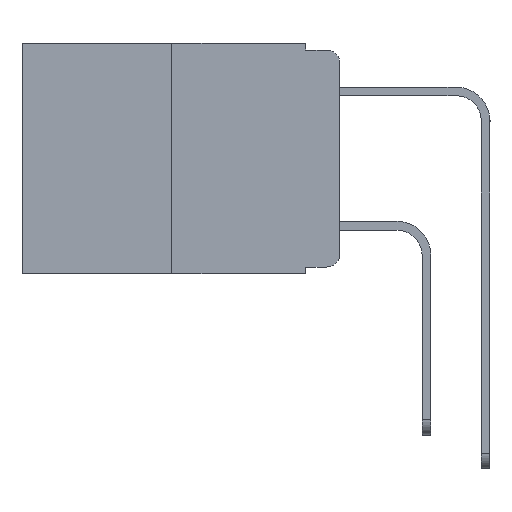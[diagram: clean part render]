
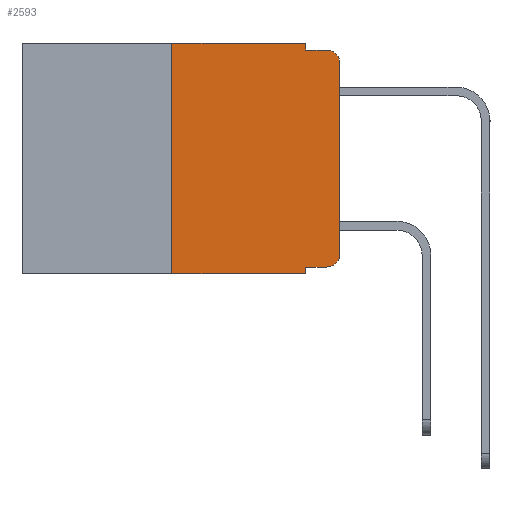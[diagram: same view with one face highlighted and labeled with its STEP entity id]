
A CAD part, left-side view. The second image highlights one B-rep face of the part: STEP entity #2593.
In plain terms, the highlighted planar face has unit normal (-1, 0, 0).
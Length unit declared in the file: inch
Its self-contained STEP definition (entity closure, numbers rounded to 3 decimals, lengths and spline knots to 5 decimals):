
#472 = CARTESIAN_POINT ( 'NONE',  ( 0., 0.051, 0. ) ) ;
#910 = EDGE_CURVE ( 'NONE', #5153, #4591, #5345, .T. ) ;
#1069 = VERTEX_POINT ( 'NONE', #21853 ) ;
#1688 = LINE ( 'NONE', #14134, #5685 ) ;
#1871 = CARTESIAN_POINT ( 'NONE',  ( 0., 0.25, -0.343 ) ) ;
#2239 = CARTESIAN_POINT ( 'NONE',  ( 0., 0.02, -0.313 ) ) ;
#2593 = ADVANCED_FACE ( 'NONE', ( #4491 ), #8141, .F. ) ;
#2603 = CARTESIAN_POINT ( 'NONE',  ( 0., 0.02, -0.333 ) ) ;
#2644 = VECTOR ( 'NONE', #14278, 39.37008 ) ;
#2890 = DIRECTION ( 'NONE',  ( 0., 0., -1. ) ) ;
#3186 = DIRECTION ( 'NONE',  ( 1., 0., 0. ) ) ;
#3280 = CARTESIAN_POINT ( 'NONE',  ( 0., 0.473, 0. ) ) ;
#3556 = DIRECTION ( 'NONE',  ( 0., -1., 0. ) ) ;
#3563 = EDGE_CURVE ( 'NONE', #10278, #11799, #20901, .T. ) ;
#3988 = DIRECTION ( 'NONE',  ( 0., 0., -1. ) ) ;
#4409 = EDGE_CURVE ( 'NONE', #4591, #10471, #15972, .T. ) ;
#4491 = FACE_OUTER_BOUND ( 'NONE', #20699, .T. ) ;
#4536 = CARTESIAN_POINT ( 'NONE',  ( 0., 0.473, -0.343 ) ) ;
#4591 = VERTEX_POINT ( 'NONE', #21033 ) ;
#5025 = CARTESIAN_POINT ( 'NONE',  ( 0., 0.02, -0.03 ) ) ;
#5153 = VERTEX_POINT ( 'NONE', #12522 ) ;
#5345 = LINE ( 'NONE', #20466, #17863 ) ;
#5370 = CARTESIAN_POINT ( 'NONE',  ( 0., 0.051, -0.01 ) ) ;
#5516 = EDGE_CURVE ( 'NONE', #16894, #10471, #6558, .T. ) ;
#5617 = CARTESIAN_POINT ( 'NONE',  ( 0., 0., -0.313 ) ) ;
#5626 = DIRECTION ( 'NONE',  ( 0., 0., 1. ) ) ;
#5685 = VECTOR ( 'NONE', #5626, 39.37008 ) ;
#6232 = VECTOR ( 'NONE', #7541, 39.37008 ) ;
#6558 = CIRCLE ( 'NONE', #13727, 0.02 ) ;
#6663 = EDGE_CURVE ( 'NONE', #15615, #16894, #15861, .T. ) ;
#6730 = DIRECTION ( 'NONE',  ( 0., 0., -1. ) ) ;
#7088 = CIRCLE ( 'NONE', #12472, 0.02 ) ;
#7541 = DIRECTION ( 'NONE',  ( 0., 0., 1. ) ) ;
#8141 = PLANE ( 'NONE',  #17940 ) ;
#8208 = LINE ( 'NONE', #13750, #17285 ) ;
#9211 = VERTEX_POINT ( 'NONE', #2603 ) ;
#9661 = DIRECTION ( 'NONE',  ( 0., -1., 0. ) ) ;
#10278 = VERTEX_POINT ( 'NONE', #1871 ) ;
#10471 = VERTEX_POINT ( 'NONE', #15963 ) ;
#10676 = CARTESIAN_POINT ( 'NONE',  ( 0., 0.25, 0. ) ) ;
#11799 = VERTEX_POINT ( 'NONE', #21342 ) ;
#12472 = AXIS2_PLACEMENT_3D ( 'NONE', #2239, #14167, #3988 ) ;
#12522 = CARTESIAN_POINT ( 'NONE',  ( 0., 0.051, 0. ) ) ;
#12553 = ORIENTED_EDGE ( 'NONE', *, *, #4409, .F. ) ;
#12594 = CARTESIAN_POINT ( 'NONE',  ( 0., 0.473, 0. ) ) ;
#12875 = ORIENTED_EDGE ( 'NONE', *, *, #21837, .F. ) ;
#13337 = ORIENTED_EDGE ( 'NONE', *, *, #5516, .T. ) ;
#13469 = ORIENTED_EDGE ( 'NONE', *, *, #14835, .F. ) ;
#13706 = ORIENTED_EDGE ( 'NONE', *, *, #3563, .T. ) ;
#13727 = AXIS2_PLACEMENT_3D ( 'NONE', #5025, #16941, #6730 ) ;
#13750 = CARTESIAN_POINT ( 'NONE',  ( 0., 0.051, -0.333 ) ) ;
#13885 = DIRECTION ( 'NONE',  ( 0., -1., 0. ) ) ;
#14134 = CARTESIAN_POINT ( 'NONE',  ( 0., 0.25, 0. ) ) ;
#14155 = ORIENTED_EDGE ( 'NONE', *, *, #910, .F. ) ;
#14167 = DIRECTION ( 'NONE',  ( -1., 0., 0. ) ) ;
#14266 = ORIENTED_EDGE ( 'NONE', *, *, #6663, .T. ) ;
#14278 = DIRECTION ( 'NONE',  ( 0., -1., 0. ) ) ;
#14835 = EDGE_CURVE ( 'NONE', #21823, #5153, #16225, .T. ) ;
#15436 = VECTOR ( 'NONE', #13885, 39.37008 ) ;
#15615 = VERTEX_POINT ( 'NONE', #5617 ) ;
#15625 = VECTOR ( 'NONE', #15884, 39.37008 ) ;
#15861 = LINE ( 'NONE', #16066, #6232 ) ;
#15884 = DIRECTION ( 'NONE',  ( 0., 0., -1. ) ) ;
#15963 = CARTESIAN_POINT ( 'NONE',  ( 0., 0.02, -0.01 ) ) ;
#15972 = LINE ( 'NONE', #5370, #15436 ) ;
#16066 = CARTESIAN_POINT ( 'NONE',  ( 0., 0., 0. ) ) ;
#16225 = LINE ( 'NONE', #12594, #2644 ) ;
#16232 = EDGE_CURVE ( 'NONE', #9211, #15615, #7088, .T. ) ;
#16407 = VECTOR ( 'NONE', #9661, 39.37008 ) ;
#16894 = VERTEX_POINT ( 'NONE', #17549 ) ;
#16941 = DIRECTION ( 'NONE',  ( -1., 0., 0. ) ) ;
#17285 = VECTOR ( 'NONE', #3556, 39.37008 ) ;
#17362 = EDGE_CURVE ( 'NONE', #1069, #9211, #8208, .T. ) ;
#17549 = CARTESIAN_POINT ( 'NONE',  ( 0., 0., -0.03 ) ) ;
#17863 = VECTOR ( 'NONE', #2890, 39.37008 ) ;
#17940 = AXIS2_PLACEMENT_3D ( 'NONE', #3280, #3186, #21511 ) ;
#18204 = ORIENTED_EDGE ( 'NONE', *, *, #20751, .F. ) ;
#20466 = CARTESIAN_POINT ( 'NONE',  ( 0., 0.051, 0. ) ) ;
#20636 = LINE ( 'NONE', #472, #15625 ) ;
#20699 = EDGE_LOOP ( 'NONE', ( #14266, #13337, #12553, #14155, #13469, #12875, #13706, #18204, #21044, #21859 ) ) ;
#20751 = EDGE_CURVE ( 'NONE', #1069, #11799, #20636, .T. ) ;
#20901 = LINE ( 'NONE', #4536, #16407 ) ;
#21033 = CARTESIAN_POINT ( 'NONE',  ( 0., 0.051, -0.01 ) ) ;
#21044 = ORIENTED_EDGE ( 'NONE', *, *, #17362, .T. ) ;
#21342 = CARTESIAN_POINT ( 'NONE',  ( 0., 0.051, -0.343 ) ) ;
#21511 = DIRECTION ( 'NONE',  ( 0., 0., -1. ) ) ;
#21823 = VERTEX_POINT ( 'NONE', #10676 ) ;
#21837 = EDGE_CURVE ( 'NONE', #10278, #21823, #1688, .T. ) ;
#21853 = CARTESIAN_POINT ( 'NONE',  ( 0., 0.051, -0.333 ) ) ;
#21859 = ORIENTED_EDGE ( 'NONE', *, *, #16232, .T. ) ;
